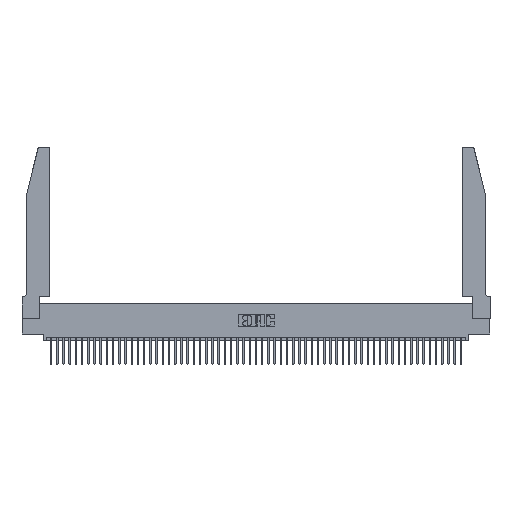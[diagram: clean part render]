
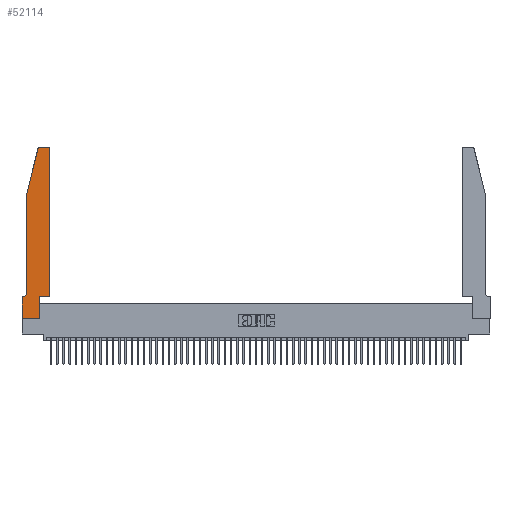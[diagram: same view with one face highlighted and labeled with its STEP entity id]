
A CAD part, top view. The second image highlights one B-rep face of the part: STEP entity #52114.
In plain terms, the highlighted planar face has unit normal (0, 0, 1).
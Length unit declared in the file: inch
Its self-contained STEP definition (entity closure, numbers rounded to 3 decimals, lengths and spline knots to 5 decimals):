
#216 = DIRECTION ( 'NONE',  ( 0., -1., 0. ) ) ;
#404 = VERTEX_POINT ( 'NONE', #15620 ) ;
#690 = ORIENTED_EDGE ( 'NONE', *, *, #50517, .T. ) ;
#2805 = ORIENTED_EDGE ( 'NONE', *, *, #44202, .T. ) ;
#2900 = VERTEX_POINT ( 'NONE', #14866 ) ;
#3297 = ORIENTED_EDGE ( 'NONE', *, *, #18139, .T. ) ;
#3492 = VERTEX_POINT ( 'NONE', #53577 ) ;
#3940 = DIRECTION ( 'NONE',  ( 0., 1., 0. ) ) ;
#4073 = VERTEX_POINT ( 'NONE', #10520 ) ;
#4143 = EDGE_CURVE ( 'NONE', #3492, #24817, #29825, .T. ) ;
#4206 = VECTOR ( 'NONE', #49329, 39.37008 ) ;
#4972 = CARTESIAN_POINT ( 'NONE',  ( 0.0755, 0.35, 0.37 ) ) ;
#5866 = VERTEX_POINT ( 'NONE', #37776 ) ;
#5993 = ORIENTED_EDGE ( 'NONE', *, *, #44620, .T. ) ;
#6067 = AXIS2_PLACEMENT_3D ( 'NONE', #50573, #16726, #46133 ) ;
#7282 = LINE ( 'NONE', #35244, #53817 ) ;
#7315 = VERTEX_POINT ( 'NONE', #22329 ) ;
#7398 = DIRECTION ( 'NONE',  ( 1., 0., 0. ) ) ;
#8322 = CARTESIAN_POINT ( 'NONE',  ( 0.4205, 2.72, 0.37 ) ) ;
#8870 = ORIENTED_EDGE ( 'NONE', *, *, #20842, .T. ) ;
#9196 = CARTESIAN_POINT ( 'NONE',  ( 0.2865, 0.35, 0.37 ) ) ;
#10291 = EDGE_CURVE ( 'NONE', #15461, #5866, #37515, .T. ) ;
#10520 = CARTESIAN_POINT ( 'NONE',  ( 0.2865, 0.35, 0.37 ) ) ;
#11751 = LINE ( 'NONE', #4972, #50402 ) ;
#13705 = DIRECTION ( 'NONE',  ( -1., 0., 0. ) ) ;
#14866 = CARTESIAN_POINT ( 'NONE',  ( 0.284, 2.75, 0.37 ) ) ;
#15461 = VERTEX_POINT ( 'NONE', #36069 ) ;
#15620 = CARTESIAN_POINT ( 'NONE',  ( 0.25487, 2.72718, 0.37 ) ) ;
#15716 = EDGE_CURVE ( 'NONE', #25827, #7315, #45141, .T. ) ;
#16726 = DIRECTION ( 'NONE',  ( 0., 0., 1. ) ) ;
#17284 = CARTESIAN_POINT ( 'NONE',  ( 0.4505, 0.35, 0.37 ) ) ;
#17644 = CARTESIAN_POINT ( 'NONE',  ( 0.0755, 2., 0.37 ) ) ;
#18139 = EDGE_CURVE ( 'NONE', #2900, #404, #44322, .T. ) ;
#18263 = LINE ( 'NONE', #33802, #50357 ) ;
#19500 = EDGE_CURVE ( 'NONE', #21668, #3492, #36760, .T. ) ;
#19774 = VECTOR ( 'NONE', #216, 39.37008 ) ;
#20809 = CARTESIAN_POINT ( 'NONE',  ( 0.2865, 0., 0.37 ) ) ;
#20842 = EDGE_CURVE ( 'NONE', #7315, #21668, #11751, .T. ) ;
#20931 = FACE_OUTER_BOUND ( 'NONE', #35184, .T. ) ;
#21213 = DIRECTION ( 'NONE',  ( -1., 0., 0. ) ) ;
#21668 = VERTEX_POINT ( 'NONE', #26829 ) ;
#22329 = CARTESIAN_POINT ( 'NONE',  ( 0.0055, 0.35, 0.37 ) ) ;
#22631 = DIRECTION ( 'NONE',  ( 0., -1., 0. ) ) ;
#23227 = CIRCLE ( 'NONE', #39191, 0.03 ) ;
#23630 = CARTESIAN_POINT ( 'NONE',  ( 0.0755, 0.42, 0.37 ) ) ;
#24534 = AXIS2_PLACEMENT_3D ( 'NONE', #25416, #25243, #21213 ) ;
#24817 = VERTEX_POINT ( 'NONE', #20809 ) ;
#25160 = CARTESIAN_POINT ( 'NONE',  ( 0., 0., 0.37 ) ) ;
#25243 = DIRECTION ( 'NONE',  ( 0., 0., -1. ) ) ;
#25416 = CARTESIAN_POINT ( 'NONE',  ( 0.0055, 0.42, 0.37 ) ) ;
#25827 = VERTEX_POINT ( 'NONE', #23630 ) ;
#26829 = CARTESIAN_POINT ( 'NONE',  ( 0., 0.35, 0.37 ) ) ;
#27807 = VERTEX_POINT ( 'NONE', #17644 ) ;
#27879 = ORIENTED_EDGE ( 'NONE', *, *, #47844, .T. ) ;
#28799 = VECTOR ( 'NONE', #44407, 39.37008 ) ;
#29825 = LINE ( 'NONE', #53515, #46852 ) ;
#31994 = CARTESIAN_POINT ( 'NONE',  ( 0.2605, 2.75, 0.37 ) ) ;
#33802 = CARTESIAN_POINT ( 'NONE',  ( 0.0755, 2., 0.37 ) ) ;
#34311 = AXIS2_PLACEMENT_3D ( 'NONE', #50812, #46733, #46542 ) ;
#35184 = EDGE_LOOP ( 'NONE', ( #27879, #3297, #51017, #2805, #40387, #8870, #35449, #39019, #690, #5993, #50953, #42588 ) ) ;
#35244 = CARTESIAN_POINT ( 'NONE',  ( 0.0755, 2., 0.37 ) ) ;
#35449 = ORIENTED_EDGE ( 'NONE', *, *, #19500, .T. ) ;
#36069 = CARTESIAN_POINT ( 'NONE',  ( 0.4505, 0.35, 0.37 ) ) ;
#36482 = CARTESIAN_POINT ( 'NONE',  ( 0.4505, 0.35, 0.37 ) ) ;
#36760 = LINE ( 'NONE', #25160, #19774 ) ;
#37489 = EDGE_CURVE ( 'NONE', #5866, #50115, #23227, .T. ) ;
#37515 = LINE ( 'NONE', #36482, #4206 ) ;
#37776 = CARTESIAN_POINT ( 'NONE',  ( 0.4505, 2.72, 0.37 ) ) ;
#37913 = DIRECTION ( 'NONE',  ( 1., 0., 0. ) ) ;
#37982 = DIRECTION ( 'NONE',  ( -0.239, -0.971, 0. ) ) ;
#38301 = PLANE ( 'NONE',  #34311 ) ;
#39019 = ORIENTED_EDGE ( 'NONE', *, *, #4143, .T. ) ;
#39191 = AXIS2_PLACEMENT_3D ( 'NONE', #8322, #41550, #45230 ) ;
#40387 = ORIENTED_EDGE ( 'NONE', *, *, #15716, .T. ) ;
#41251 = LINE ( 'NONE', #31994, #28799 ) ;
#41550 = DIRECTION ( 'NONE',  ( 0., 0., 1. ) ) ;
#42233 = VECTOR ( 'NONE', #3940, 39.37008 ) ;
#42588 = ORIENTED_EDGE ( 'NONE', *, *, #37489, .T. ) ;
#43577 = LINE ( 'NONE', #9196, #42233 ) ;
#44202 = EDGE_CURVE ( 'NONE', #27807, #25827, #7282, .T. ) ;
#44322 = CIRCLE ( 'NONE', #6067, 0.03 ) ;
#44407 = DIRECTION ( 'NONE',  ( -1., 0., 0. ) ) ;
#44620 = EDGE_CURVE ( 'NONE', #4073, #15461, #51755, .T. ) ;
#45141 = CIRCLE ( 'NONE', #24534, 0.07 ) ;
#45230 = DIRECTION ( 'NONE',  ( 1., 0., 0. ) ) ;
#46133 = DIRECTION ( 'NONE',  ( 1., 0., 0. ) ) ;
#46542 = DIRECTION ( 'NONE',  ( 1., 0., 0. ) ) ;
#46733 = DIRECTION ( 'NONE',  ( 0., 0., 1. ) ) ;
#46852 = VECTOR ( 'NONE', #7398, 39.37008 ) ;
#47449 = CARTESIAN_POINT ( 'NONE',  ( 0.4205, 2.75, 0.37 ) ) ;
#47844 = EDGE_CURVE ( 'NONE', #50115, #2900, #41251, .T. ) ;
#49169 = EDGE_CURVE ( 'NONE', #404, #27807, #18263, .T. ) ;
#49329 = DIRECTION ( 'NONE',  ( 0., 1., 0. ) ) ;
#50115 = VERTEX_POINT ( 'NONE', #47449 ) ;
#50357 = VECTOR ( 'NONE', #37982, 39.37008 ) ;
#50402 = VECTOR ( 'NONE', #13705, 39.37008 ) ;
#50517 = EDGE_CURVE ( 'NONE', #24817, #4073, #43577, .T. ) ;
#50573 = CARTESIAN_POINT ( 'NONE',  ( 0.284, 2.72, 0.37 ) ) ;
#50812 = CARTESIAN_POINT ( 'NONE',  ( 0., 0.35, 0.37 ) ) ;
#50953 = ORIENTED_EDGE ( 'NONE', *, *, #10291, .T. ) ;
#51017 = ORIENTED_EDGE ( 'NONE', *, *, #49169, .T. ) ;
#51101 = VECTOR ( 'NONE', #37913, 39.37008 ) ;
#51755 = LINE ( 'NONE', #17284, #51101 ) ;
#52114 = ADVANCED_FACE ( 'NONE', ( #20931 ), #38301, .T. ) ;
#53515 = CARTESIAN_POINT ( 'NONE',  ( 0., 0., 0.37 ) ) ;
#53577 = CARTESIAN_POINT ( 'NONE',  ( 0., 0., 0.37 ) ) ;
#53817 = VECTOR ( 'NONE', #22631, 39.37008 ) ;
